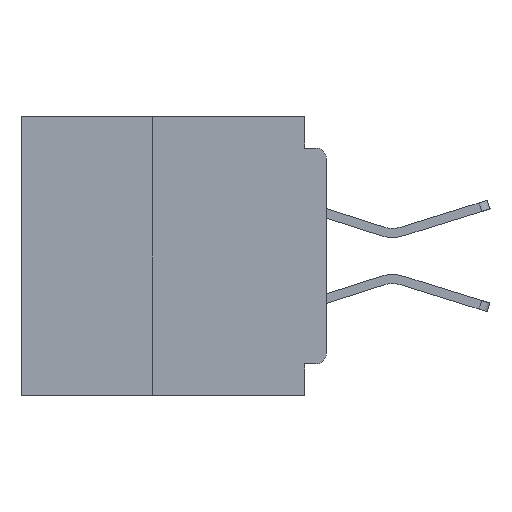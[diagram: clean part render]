
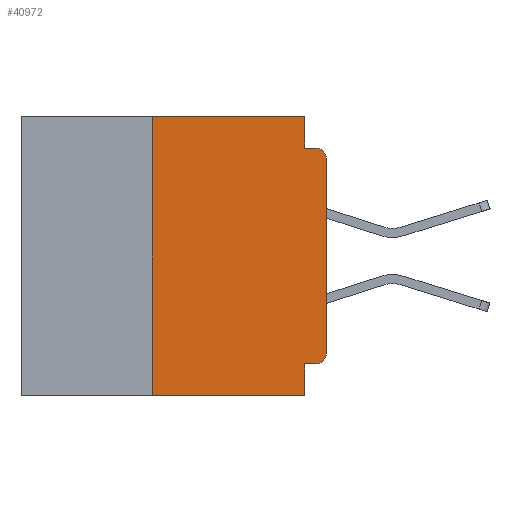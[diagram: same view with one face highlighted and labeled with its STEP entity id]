
A CAD part, left-side view. The second image highlights one B-rep face of the part: STEP entity #40972.
In plain terms, the highlighted planar face has unit normal (-1, 0, 0).
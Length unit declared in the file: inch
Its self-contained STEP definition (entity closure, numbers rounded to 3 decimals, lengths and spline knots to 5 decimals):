
#293 = DIRECTION ( 'NONE',  ( -1., 0., 0. ) ) ;
#1228 = DIRECTION ( 'NONE',  ( 0., 0., -1. ) ) ;
#2222 = VECTOR ( 'NONE', #4860, 39.37008 ) ;
#3939 = CARTESIAN_POINT ( 'NONE',  ( 0., 0.25, 0. ) ) ;
#4523 = DIRECTION ( 'NONE',  ( 0., -1., 0. ) ) ;
#4770 = DIRECTION ( 'NONE',  ( 0., 0., 1. ) ) ;
#4860 = DIRECTION ( 'NONE',  ( 0., 1., 0. ) ) ;
#5042 = DIRECTION ( 'NONE',  ( 0., 0., 1. ) ) ;
#6949 = VECTOR ( 'NONE', #31770, 39.37008 ) ;
#7110 = ORIENTED_EDGE ( 'NONE', *, *, #59494, .T. ) ;
#7455 = CARTESIAN_POINT ( 'NONE',  ( 0., 0.437, 0. ) ) ;
#8514 = CIRCLE ( 'NONE', #24647, 0.015 ) ;
#10544 = VERTEX_POINT ( 'NONE', #43739 ) ;
#10561 = EDGE_CURVE ( 'NONE', #11305, #24968, #39923, .T. ) ;
#11305 = VERTEX_POINT ( 'NONE', #15913 ) ;
#11764 = ORIENTED_EDGE ( 'NONE', *, *, #22338, .F. ) ;
#13016 = DIRECTION ( 'NONE',  ( 0., -1., 0. ) ) ;
#13361 = ORIENTED_EDGE ( 'NONE', *, *, #51103, .F. ) ;
#15913 = CARTESIAN_POINT ( 'NONE',  ( 0., 0., -0.06 ) ) ;
#16070 = VECTOR ( 'NONE', #13016, 39.37008 ) ;
#17456 = EDGE_CURVE ( 'NONE', #37589, #35761, #61153, .T. ) ;
#17533 = LINE ( 'NONE', #48762, #53129 ) ;
#17775 = ORIENTED_EDGE ( 'NONE', *, *, #36775, .F. ) ;
#19115 = VERTEX_POINT ( 'NONE', #53029 ) ;
#19558 = PLANE ( 'NONE',  #50404 ) ;
#19748 = EDGE_CURVE ( 'NONE', #28474, #54536, #30811, .T. ) ;
#21083 = VECTOR ( 'NONE', #5042, 39.37008 ) ;
#22203 = DIRECTION ( 'NONE',  ( 0., -1., 0. ) ) ;
#22338 = EDGE_CURVE ( 'NONE', #54308, #54536, #17533, .T. ) ;
#23997 = CARTESIAN_POINT ( 'NONE',  ( 0., 0.437, -0.4 ) ) ;
#24177 = CARTESIAN_POINT ( 'NONE',  ( 0., 0.031, -0.045 ) ) ;
#24647 = AXIS2_PLACEMENT_3D ( 'NONE', #59404, #30493, #1228 ) ;
#24671 = DIRECTION ( 'NONE',  ( 0., 0., -1. ) ) ;
#24968 = VERTEX_POINT ( 'NONE', #34780 ) ;
#26944 = CARTESIAN_POINT ( 'NONE',  ( 0., 0.031, 0. ) ) ;
#28474 = VERTEX_POINT ( 'NONE', #62542 ) ;
#29322 = DIRECTION ( 'NONE',  ( 0., 0., -1. ) ) ;
#29571 = CARTESIAN_POINT ( 'NONE',  ( 0., 0.015, -0.06 ) ) ;
#30493 = DIRECTION ( 'NONE',  ( -1., 0., 0. ) ) ;
#30811 = LINE ( 'NONE', #23997, #56483 ) ;
#31341 = LINE ( 'NONE', #26944, #6949 ) ;
#31770 = DIRECTION ( 'NONE',  ( 0., 0., -1. ) ) ;
#32254 = ORIENTED_EDGE ( 'NONE', *, *, #10561, .T. ) ;
#34225 = CARTESIAN_POINT ( 'NONE',  ( 0., 0., 0. ) ) ;
#34419 = DIRECTION ( 'NONE',  ( 0., 0., -1. ) ) ;
#34556 = FACE_OUTER_BOUND ( 'NONE', #42030, .T. ) ;
#34780 = CARTESIAN_POINT ( 'NONE',  ( 0., 0.015, -0.045 ) ) ;
#35761 = VERTEX_POINT ( 'NONE', #42653 ) ;
#36775 = EDGE_CURVE ( 'NONE', #35761, #45143, #31341, .T. ) ;
#37184 = CARTESIAN_POINT ( 'NONE',  ( 0., 0., -0.045 ) ) ;
#37490 = EDGE_CURVE ( 'NONE', #45143, #24968, #41825, .T. ) ;
#37589 = VERTEX_POINT ( 'NONE', #3939 ) ;
#39923 = CIRCLE ( 'NONE', #41119, 0.015 ) ;
#40972 = ADVANCED_FACE ( 'NONE', ( #34556 ), #19558, .F. ) ;
#41119 = AXIS2_PLACEMENT_3D ( 'NONE', #29571, #293, #34419 ) ;
#41825 = LINE ( 'NONE', #37184, #16070 ) ;
#42030 = EDGE_LOOP ( 'NONE', ( #7110, #32254, #61383, #17775, #57059, #13361, #45206, #11764, #51381, #51362 ) ) ;
#42653 = CARTESIAN_POINT ( 'NONE',  ( 0., 0.031, 0. ) ) ;
#43739 = CARTESIAN_POINT ( 'NONE',  ( 0., 0.015, -0.355 ) ) ;
#45143 = VERTEX_POINT ( 'NONE', #24177 ) ;
#45206 = ORIENTED_EDGE ( 'NONE', *, *, #19748, .T. ) ;
#48557 = CARTESIAN_POINT ( 'NONE',  ( 0., 0.25, -0.4 ) ) ;
#48762 = CARTESIAN_POINT ( 'NONE',  ( 0., 0.031, -0.4 ) ) ;
#50404 = AXIS2_PLACEMENT_3D ( 'NONE', #53414, #58252, #29322 ) ;
#51103 = EDGE_CURVE ( 'NONE', #28474, #37589, #60869, .T. ) ;
#51362 = ORIENTED_EDGE ( 'NONE', *, *, #55893, .T. ) ;
#51381 = ORIENTED_EDGE ( 'NONE', *, *, #52327, .F. ) ;
#52327 = EDGE_CURVE ( 'NONE', #10544, #54308, #55452, .T. ) ;
#53029 = CARTESIAN_POINT ( 'NONE',  ( 0., 0., -0.34 ) ) ;
#53129 = VECTOR ( 'NONE', #24671, 39.37008 ) ;
#53414 = CARTESIAN_POINT ( 'NONE',  ( 0., 0.437, 0. ) ) ;
#53500 = CARTESIAN_POINT ( 'NONE',  ( 0., 0., -0.355 ) ) ;
#54308 = VERTEX_POINT ( 'NONE', #57643 ) ;
#54536 = VERTEX_POINT ( 'NONE', #60359 ) ;
#55119 = VECTOR ( 'NONE', #22203, 39.37008 ) ;
#55452 = LINE ( 'NONE', #53500, #2222 ) ;
#55893 = EDGE_CURVE ( 'NONE', #10544, #19115, #8514, .T. ) ;
#56483 = VECTOR ( 'NONE', #4523, 39.37008 ) ;
#57059 = ORIENTED_EDGE ( 'NONE', *, *, #17456, .F. ) ;
#57643 = CARTESIAN_POINT ( 'NONE',  ( 0., 0.031, -0.355 ) ) ;
#58145 = LINE ( 'NONE', #34225, #21083 ) ;
#58252 = DIRECTION ( 'NONE',  ( 1., 0., 0. ) ) ;
#59369 = VECTOR ( 'NONE', #4770, 39.37008 ) ;
#59404 = CARTESIAN_POINT ( 'NONE',  ( 0., 0.015, -0.34 ) ) ;
#59494 = EDGE_CURVE ( 'NONE', #19115, #11305, #58145, .T. ) ;
#60359 = CARTESIAN_POINT ( 'NONE',  ( 0., 0.031, -0.4 ) ) ;
#60869 = LINE ( 'NONE', #48557, #59369 ) ;
#61153 = LINE ( 'NONE', #7455, #55119 ) ;
#61383 = ORIENTED_EDGE ( 'NONE', *, *, #37490, .F. ) ;
#62542 = CARTESIAN_POINT ( 'NONE',  ( 0., 0.25, -0.4 ) ) ;
